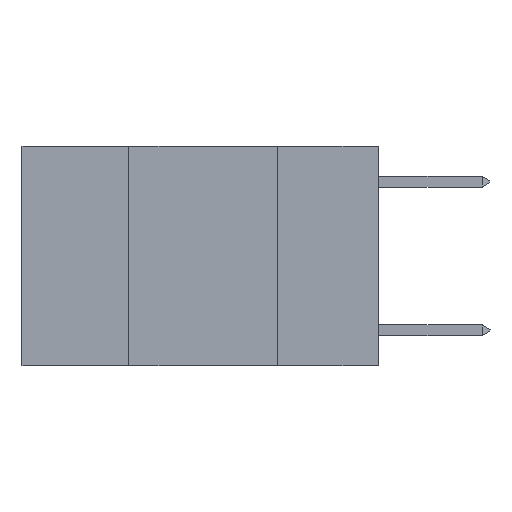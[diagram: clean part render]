
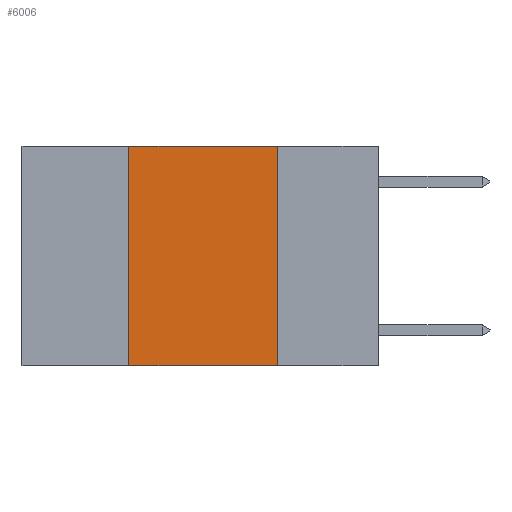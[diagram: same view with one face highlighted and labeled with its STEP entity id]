
A CAD part, left-side view. The second image highlights one B-rep face of the part: STEP entity #6006.
In plain terms, the highlighted planar face has unit normal (-1, 0, 0).
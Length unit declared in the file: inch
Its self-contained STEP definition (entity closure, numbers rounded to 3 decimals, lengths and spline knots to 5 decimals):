
#398 = ORIENTED_EDGE ( 'NONE', *, *, #16300, .F. ) ;
#777 = CARTESIAN_POINT ( 'NONE',  ( 0., 0.17, 0. ) ) ;
#2483 = DIRECTION ( 'NONE',  ( 0., -1., 0. ) ) ;
#2502 = DIRECTION ( 'NONE',  ( 0., -1., 0. ) ) ;
#2559 = CARTESIAN_POINT ( 'NONE',  ( 0., 0.6, -0.37 ) ) ;
#2803 = CARTESIAN_POINT ( 'NONE',  ( 0., 0.6, 0. ) ) ;
#4041 = ORIENTED_EDGE ( 'NONE', *, *, #13843, .F. ) ;
#4616 = DIRECTION ( 'NONE',  ( 0., 0., 1. ) ) ;
#4687 = VECTOR ( 'NONE', #4616, 39.37008 ) ;
#4807 = LINE ( 'NONE', #4876, #4687 ) ;
#4876 = CARTESIAN_POINT ( 'NONE',  ( 0., 0.42, 0. ) ) ;
#6006 = ADVANCED_FACE ( 'NONE', ( #14246 ), #21149, .F. ) ;
#6733 = VECTOR ( 'NONE', #2502, 39.37008 ) ;
#6775 = LINE ( 'NONE', #2803, #6733 ) ;
#6933 = VERTEX_POINT ( 'NONE', #18679 ) ;
#7651 = VECTOR ( 'NONE', #12818, 39.37008 ) ;
#7918 = LINE ( 'NONE', #14095, #7651 ) ;
#8291 = EDGE_LOOP ( 'NONE', ( #4041, #398, #21053, #15109 ) ) ;
#8340 = AXIS2_PLACEMENT_3D ( 'NONE', #20811, #20610, #20757 ) ;
#8419 = CARTESIAN_POINT ( 'NONE',  ( 0., 0.17, -0.37 ) ) ;
#10422 = EDGE_CURVE ( 'NONE', #6933, #21525, #10988, .T. ) ;
#10886 = VECTOR ( 'NONE', #2483, 39.37008 ) ;
#10988 = LINE ( 'NONE', #2559, #10886 ) ;
#11585 = EDGE_CURVE ( 'NONE', #6933, #12453, #4807, .T. ) ;
#12453 = VERTEX_POINT ( 'NONE', #16325 ) ;
#12818 = DIRECTION ( 'NONE',  ( 0., 0., -1. ) ) ;
#13843 = EDGE_CURVE ( 'NONE', #17656, #21525, #7918, .T. ) ;
#14095 = CARTESIAN_POINT ( 'NONE',  ( 0., 0.17, 0. ) ) ;
#14246 = FACE_OUTER_BOUND ( 'NONE', #8291, .T. ) ;
#15109 = ORIENTED_EDGE ( 'NONE', *, *, #10422, .T. ) ;
#16300 = EDGE_CURVE ( 'NONE', #12453, #17656, #6775, .T. ) ;
#16325 = CARTESIAN_POINT ( 'NONE',  ( 0., 0.42, 0. ) ) ;
#17656 = VERTEX_POINT ( 'NONE', #777 ) ;
#18679 = CARTESIAN_POINT ( 'NONE',  ( 0., 0.42, -0.37 ) ) ;
#20610 = DIRECTION ( 'NONE',  ( 1., 0., 0. ) ) ;
#20757 = DIRECTION ( 'NONE',  ( 0., 0., -1. ) ) ;
#20811 = CARTESIAN_POINT ( 'NONE',  ( 0., 0.6, 0. ) ) ;
#21053 = ORIENTED_EDGE ( 'NONE', *, *, #11585, .F. ) ;
#21149 = PLANE ( 'NONE',  #8340 ) ;
#21525 = VERTEX_POINT ( 'NONE', #8419 ) ;
